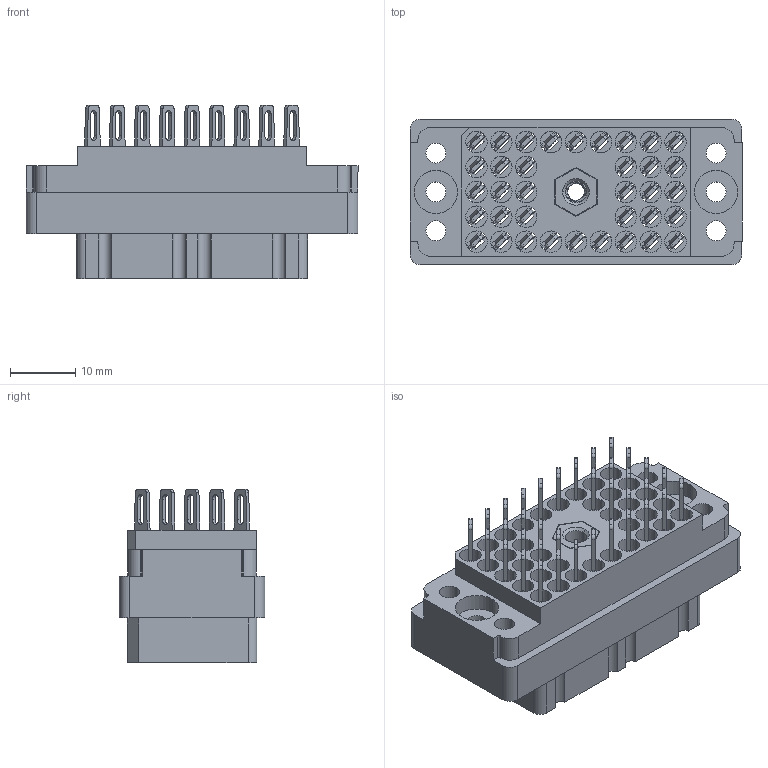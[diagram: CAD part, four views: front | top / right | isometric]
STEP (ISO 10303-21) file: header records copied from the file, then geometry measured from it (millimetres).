
FILE_DESCRIPTION (( 'STEP AP203' ), '1' );
FILE_NAME ('519-036-500-406.STEP', '2020-09-09T20:14:38', ( '' ), ( '' ), 'SwSTEP 2.0', 'SolidWorks 2020', '' );
FILE_SCHEMA (( 'CONFIG_CONTROL_DESIGN' ));
Length unit declared in the file: inch
Products named in the file (4): 519-036-500-406; 516-292-001_500 Contact; 516-252-035-100_516-252-035-100; 519 Receptacle Insulator_036
Assembly tree (38 placements, depth 2):
  519-036-500-406
    519 Receptacle Insulator_036
    516-292-001_500 Contact  x36
    516-252-035-100_516-252-035-100
Bounding box: 50.8 x 22.25 x 26.49 mm (x, y, z)
Volume: 12576.5 mm3; surface area: 20962.4 mm2
Topology: 38 solids, 38 shells, 3636 faces, 10541 edges, 7000 vertices
Faces by surface type: plane 2170, cylinder 1232, bspline 222, cone 12
Entity records: 36436 total; most frequent: CARTESIAN_POINT 8479, ORIENTED_EDGE 5682, DIRECTION 5465, EDGE_CURVE 2841, VECTOR 2059, LINE 2059, VERTEX_POINT 1890, AXIS2_PLACEMENT_3D 1703
